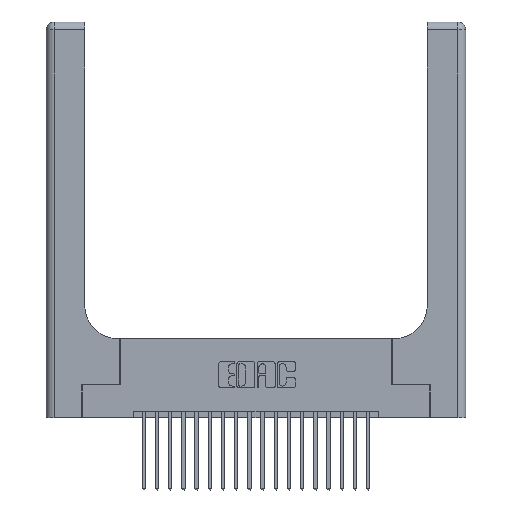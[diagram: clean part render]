
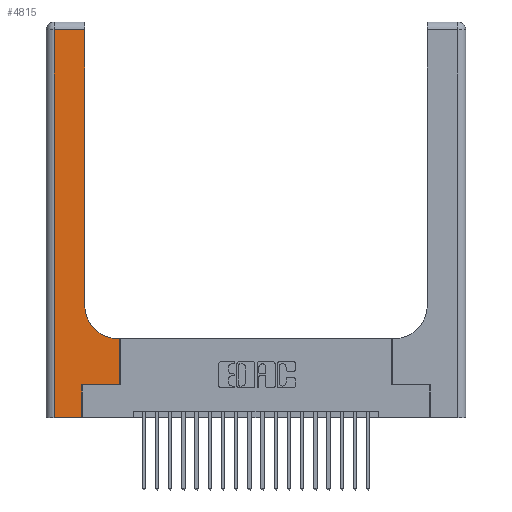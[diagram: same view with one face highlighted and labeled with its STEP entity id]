
A CAD part, top view. The second image highlights one B-rep face of the part: STEP entity #4815.
In plain terms, the highlighted planar face has unit normal (0, 0, 1).
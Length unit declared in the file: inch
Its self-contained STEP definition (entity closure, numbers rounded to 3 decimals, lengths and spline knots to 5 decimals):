
#46 = LINE ( 'NONE', #21817, #8880 ) ;
#702 = VERTEX_POINT ( 'NONE', #7693 ) ;
#980 = AXIS2_PLACEMENT_3D ( 'NONE', #9502, #21574, #11255 ) ;
#1475 = VECTOR ( 'NONE', #11181, 39.37008 ) ;
#1501 = FACE_OUTER_BOUND ( 'NONE', #20985, .T. ) ;
#1831 = VECTOR ( 'NONE', #4960, 39.37008 ) ;
#3149 = DIRECTION ( 'NONE',  ( 0., -1., 0. ) ) ;
#3157 = CARTESIAN_POINT ( 'NONE',  ( 0.269, 0., 0.37 ) ) ;
#3467 = ORIENTED_EDGE ( 'NONE', *, *, #8404, .T. ) ;
#3734 = VECTOR ( 'NONE', #22355, 39.37008 ) ;
#4067 = VERTEX_POINT ( 'NONE', #12775 ) ;
#4168 = VECTOR ( 'NONE', #21380, 39.37008 ) ;
#4815 = ADVANCED_FACE ( 'NONE', ( #1501 ), #16815, .F. ) ;
#4842 = VERTEX_POINT ( 'NONE', #15344 ) ;
#4915 = CARTESIAN_POINT ( 'NONE',  ( 0.269, 0.25, 0.37 ) ) ;
#4960 = DIRECTION ( 'NONE',  ( 1., 0., 0. ) ) ;
#5706 = ORIENTED_EDGE ( 'NONE', *, *, #11114, .T. ) ;
#5960 = VECTOR ( 'NONE', #3149, 39.37008 ) ;
#6356 = DIRECTION ( 'NONE',  ( 0., 0., -1. ) ) ;
#7101 = CARTESIAN_POINT ( 'NONE',  ( 0.5415, 0.6, 0.37 ) ) ;
#7188 = CARTESIAN_POINT ( 'NONE',  ( 0.2915, 3., 0.37 ) ) ;
#7512 = CARTESIAN_POINT ( 'NONE',  ( 0.5585, 0.25, 0.37 ) ) ;
#7693 = CARTESIAN_POINT ( 'NONE',  ( 0.5585, 0.6, 0.37 ) ) ;
#7879 = VECTOR ( 'NONE', #13791, 39.37008 ) ;
#8196 = EDGE_CURVE ( 'NONE', #14152, #14448, #10663, .T. ) ;
#8404 = EDGE_CURVE ( 'NONE', #12813, #4842, #20119, .T. ) ;
#8471 = LINE ( 'NONE', #3157, #3734 ) ;
#8880 = VECTOR ( 'NONE', #16719, 39.37008 ) ;
#9029 = VERTEX_POINT ( 'NONE', #12570 ) ;
#9200 = EDGE_CURVE ( 'NONE', #10738, #12813, #14170, .T. ) ;
#9502 = CARTESIAN_POINT ( 'NONE',  ( 0.5415, 0.85, 0.37 ) ) ;
#9853 = CARTESIAN_POINT ( 'NONE',  ( 0., 3., 0.37 ) ) ;
#10663 = LINE ( 'NONE', #17192, #1831 ) ;
#10679 = DIRECTION ( 'NONE',  ( 0., 1., 0. ) ) ;
#10738 = VERTEX_POINT ( 'NONE', #7101 ) ;
#11114 = EDGE_CURVE ( 'NONE', #4842, #4067, #46, .T. ) ;
#11181 = DIRECTION ( 'NONE',  ( -1., 0., 0. ) ) ;
#11255 = DIRECTION ( 'NONE',  ( 1., 0., 0. ) ) ;
#11474 = VECTOR ( 'NONE', #10679, 39.37008 ) ;
#11968 = CARTESIAN_POINT ( 'NONE',  ( 0.06, 3., 0.37 ) ) ;
#12570 = CARTESIAN_POINT ( 'NONE',  ( 0.5585, 0.25, 0.37 ) ) ;
#12775 = CARTESIAN_POINT ( 'NONE',  ( 0.06, 2.94, 0.37 ) ) ;
#12813 = VERTEX_POINT ( 'NONE', #12877 ) ;
#12877 = CARTESIAN_POINT ( 'NONE',  ( 0.2915, 0.85, 0.37 ) ) ;
#13548 = CARTESIAN_POINT ( 'NONE',  ( 0.06, 0., 0.37 ) ) ;
#13618 = ORIENTED_EDGE ( 'NONE', *, *, #21257, .T. ) ;
#13657 = ORIENTED_EDGE ( 'NONE', *, *, #18909, .T. ) ;
#13791 = DIRECTION ( 'NONE',  ( 1., 0., 0. ) ) ;
#14152 = VERTEX_POINT ( 'NONE', #13548 ) ;
#14170 = CIRCLE ( 'NONE', #980, 0.25 ) ;
#14286 = CARTESIAN_POINT ( 'NONE',  ( 0.269, 0., 0.37 ) ) ;
#14448 = VERTEX_POINT ( 'NONE', #14286 ) ;
#14456 = CARTESIAN_POINT ( 'NONE',  ( 0.269, 0.25, 0.37 ) ) ;
#14830 = ORIENTED_EDGE ( 'NONE', *, *, #17349, .T. ) ;
#14877 = ORIENTED_EDGE ( 'NONE', *, *, #18405, .T. ) ;
#15138 = ORIENTED_EDGE ( 'NONE', *, *, #8196, .T. ) ;
#15344 = CARTESIAN_POINT ( 'NONE',  ( 0.2915, 2.94, 0.37 ) ) ;
#16415 = CARTESIAN_POINT ( 'NONE',  ( 0.2915, 0.6, 0.37 ) ) ;
#16719 = DIRECTION ( 'NONE',  ( -1., 0., 0. ) ) ;
#16815 = PLANE ( 'NONE',  #22524 ) ;
#17192 = CARTESIAN_POINT ( 'NONE',  ( 0., 0., 0.37 ) ) ;
#17215 = ORIENTED_EDGE ( 'NONE', *, *, #9200, .T. ) ;
#17349 = EDGE_CURVE ( 'NONE', #4067, #14152, #19868, .T. ) ;
#18131 = LINE ( 'NONE', #7512, #4168 ) ;
#18405 = EDGE_CURVE ( 'NONE', #14448, #18569, #8471, .T. ) ;
#18557 = DIRECTION ( 'NONE',  ( -1., 0., 0. ) ) ;
#18569 = VERTEX_POINT ( 'NONE', #14456 ) ;
#18570 = ORIENTED_EDGE ( 'NONE', *, *, #20465, .T. ) ;
#18909 = EDGE_CURVE ( 'NONE', #18569, #9029, #21709, .T. ) ;
#19504 = LINE ( 'NONE', #16415, #1475 ) ;
#19868 = LINE ( 'NONE', #11968, #5960 ) ;
#20119 = LINE ( 'NONE', #7188, #11474 ) ;
#20465 = EDGE_CURVE ( 'NONE', #702, #10738, #19504, .T. ) ;
#20985 = EDGE_LOOP ( 'NONE', ( #3467, #5706, #14830, #15138, #14877, #13657, #13618, #18570, #17215 ) ) ;
#21257 = EDGE_CURVE ( 'NONE', #9029, #702, #18131, .T. ) ;
#21380 = DIRECTION ( 'NONE',  ( 0., 1., 0. ) ) ;
#21574 = DIRECTION ( 'NONE',  ( 0., 0., -1. ) ) ;
#21709 = LINE ( 'NONE', #4915, #7879 ) ;
#21817 = CARTESIAN_POINT ( 'NONE',  ( 0., 2.94, 0.37 ) ) ;
#22355 = DIRECTION ( 'NONE',  ( 0., 1., 0. ) ) ;
#22524 = AXIS2_PLACEMENT_3D ( 'NONE', #9853, #6356, #18557 ) ;
